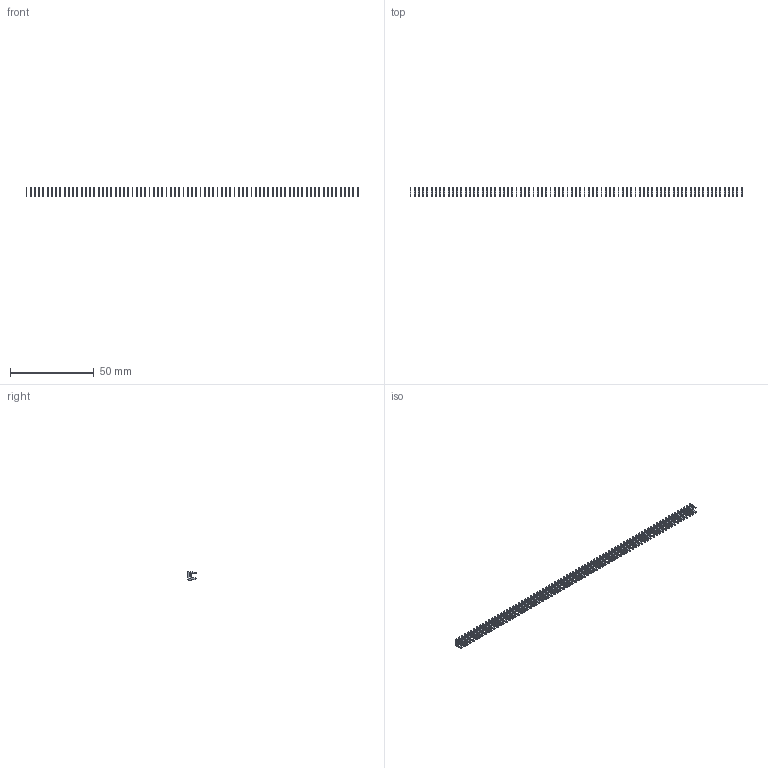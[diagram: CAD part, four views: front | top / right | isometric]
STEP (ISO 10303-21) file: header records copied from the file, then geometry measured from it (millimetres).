
FILE_DESCRIPTION (( 'STEP AP203' ), '1' );
FILE_NAME ('105-079-208-100.STEP', '2020-04-08T01:07:08', ( '' ), ( '' ), 'SwSTEP 2.0', 'SolidWorks 2016', '' );
FILE_SCHEMA (( 'CONFIG_CONTROL_DESIGN' ));
Length unit declared in the file: inch
Products named in the file (2): 105-079-208-100; 100-290-001_100-290-208
Assembly tree (79 placements, depth 2):
  105-079-208-100
    100-290-001_100-290-208  x79
Bounding box: 198.63 x 4.83 x 5.17 mm (x, y, z)
Volume: 543.6 mm3; surface area: 3357.2 mm2
Topology: 79 solids, 79 shells, 1975 faces, 5451 edges, 3634 vertices
Faces by surface type: plane 1738, cylinder 237
Entity records: 3485 total; most frequent: DIRECTION 289, CARTESIAN_POINT 222, COORDINATED_UNIVERSAL_TIME_OFFSET 168, LOCAL_TIME 168, DATE_AND_TIME 168, CALENDAR_DATE 168, ORIENTED_EDGE 138, AXIS2_PLACEMENT_3D 113
